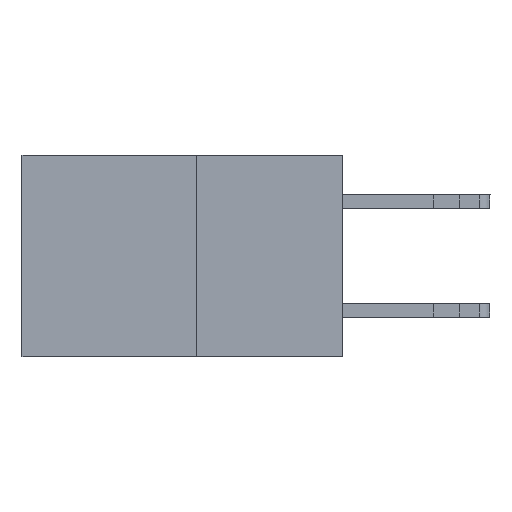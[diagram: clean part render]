
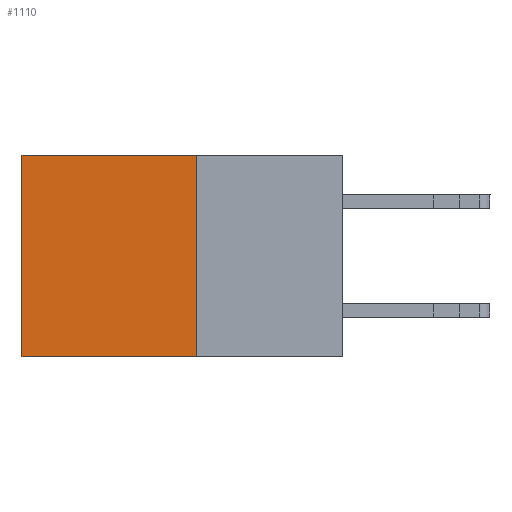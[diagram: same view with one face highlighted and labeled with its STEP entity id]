
A CAD part, left-side view. The second image highlights one B-rep face of the part: STEP entity #1110.
In plain terms, the highlighted planar face has unit normal (-1, 0, 0).
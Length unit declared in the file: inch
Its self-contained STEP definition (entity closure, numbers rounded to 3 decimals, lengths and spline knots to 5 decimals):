
#1086 = ORIENTED_EDGE ( 'NONE', *, *, #9604, .T. ) ;
#1110 = ADVANCED_FACE ( 'NONE', ( #8161 ), #4500, .F. ) ;
#1982 = EDGE_CURVE ( 'NONE', #4242, #8644, #5869, .T. ) ;
#2187 = VECTOR ( 'NONE', #8553, 39.37008 ) ;
#2626 = CARTESIAN_POINT ( 'NONE',  ( 0.277, 0.59, -0.37 ) ) ;
#2744 = AXIS2_PLACEMENT_3D ( 'NONE', #13130, #9644, #9553 ) ;
#3264 = VERTEX_POINT ( 'NONE', #12130 ) ;
#3277 = ORIENTED_EDGE ( 'NONE', *, *, #8327, .F. ) ;
#3514 = CARTESIAN_POINT ( 'NONE',  ( 0.277, 0.27, -0.37 ) ) ;
#4242 = VERTEX_POINT ( 'NONE', #13318 ) ;
#4500 = PLANE ( 'NONE',  #2744 ) ;
#4928 = LINE ( 'NONE', #6162, #6351 ) ;
#5869 = LINE ( 'NONE', #6868, #8571 ) ;
#6162 = CARTESIAN_POINT ( 'NONE',  ( 0.277, 0.59, -0.37 ) ) ;
#6351 = VECTOR ( 'NONE', #15184, 39.37008 ) ;
#6868 = CARTESIAN_POINT ( 'NONE',  ( 0.277, 0.27, 0. ) ) ;
#7186 = CARTESIAN_POINT ( 'NONE',  ( 0.277, 0.59, 0. ) ) ;
#7809 = ORIENTED_EDGE ( 'NONE', *, *, #1982, .T. ) ;
#8161 = FACE_OUTER_BOUND ( 'NONE', #12244, .T. ) ;
#8327 = EDGE_CURVE ( 'NONE', #3264, #9691, #9011, .T. ) ;
#8553 = DIRECTION ( 'NONE',  ( 0., 0., -1. ) ) ;
#8571 = VECTOR ( 'NONE', #10826, 39.37008 ) ;
#8644 = VERTEX_POINT ( 'NONE', #7186 ) ;
#9011 = LINE ( 'NONE', #10421, #10557 ) ;
#9553 = DIRECTION ( 'NONE',  ( 0., 0., -1. ) ) ;
#9604 = EDGE_CURVE ( 'NONE', #8644, #9691, #4928, .T. ) ;
#9644 = DIRECTION ( 'NONE',  ( 1., 0., 0. ) ) ;
#9691 = VERTEX_POINT ( 'NONE', #2626 ) ;
#10421 = CARTESIAN_POINT ( 'NONE',  ( 0.277, 0.27, -0.37 ) ) ;
#10557 = VECTOR ( 'NONE', #12583, 39.37008 ) ;
#10826 = DIRECTION ( 'NONE',  ( 0., 1., 0. ) ) ;
#11419 = EDGE_CURVE ( 'NONE', #4242, #3264, #13439, .T. ) ;
#12130 = CARTESIAN_POINT ( 'NONE',  ( 0.277, 0.27, -0.37 ) ) ;
#12244 = EDGE_LOOP ( 'NONE', ( #1086, #3277, #16154, #7809 ) ) ;
#12583 = DIRECTION ( 'NONE',  ( 0., 1., 0. ) ) ;
#13130 = CARTESIAN_POINT ( 'NONE',  ( 0.277, 0.27, -0.37 ) ) ;
#13318 = CARTESIAN_POINT ( 'NONE',  ( 0.277, 0.27, 0. ) ) ;
#13439 = LINE ( 'NONE', #3514, #2187 ) ;
#15184 = DIRECTION ( 'NONE',  ( 0., 0., -1. ) ) ;
#16154 = ORIENTED_EDGE ( 'NONE', *, *, #11419, .F. ) ;
